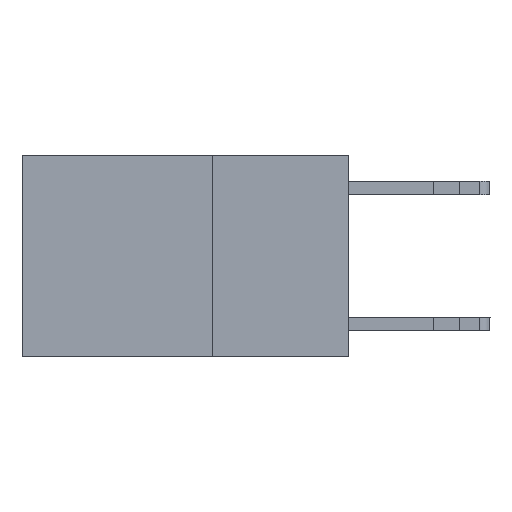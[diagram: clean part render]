
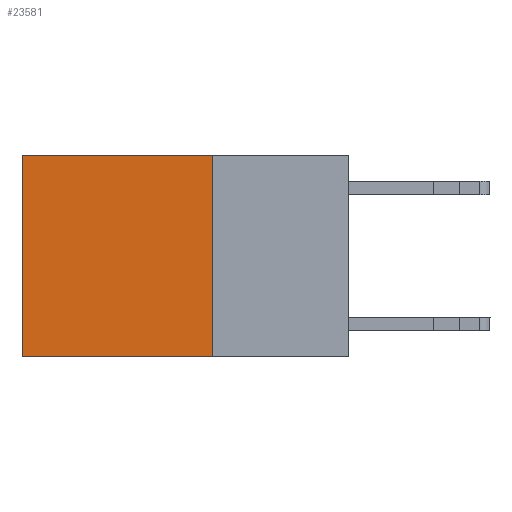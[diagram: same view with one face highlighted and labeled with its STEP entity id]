
A CAD part, left-side view. The second image highlights one B-rep face of the part: STEP entity #23581.
In plain terms, the highlighted planar face has unit normal (-1, 0, 0).
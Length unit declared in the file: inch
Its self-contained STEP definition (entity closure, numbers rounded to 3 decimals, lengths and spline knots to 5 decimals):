
#465 = EDGE_LOOP ( 'NONE', ( #22984, #8860, #528, #7988 ) ) ;
#528 = ORIENTED_EDGE ( 'NONE', *, *, #6625, .F. ) ;
#1226 = VERTEX_POINT ( 'NONE', #23646 ) ;
#1746 = FACE_OUTER_BOUND ( 'NONE', #465, .T. ) ;
#3121 = EDGE_CURVE ( 'NONE', #1226, #10511, #5561, .T. ) ;
#5373 = VECTOR ( 'NONE', #13706, 39.37008 ) ;
#5561 = LINE ( 'NONE', #11869, #5373 ) ;
#5748 = CARTESIAN_POINT ( 'NONE',  ( 0.2625, 0.6, -0.37 ) ) ;
#5767 = CARTESIAN_POINT ( 'NONE',  ( 0.2625, 0.25, 0. ) ) ;
#6070 = VECTOR ( 'NONE', #19828, 39.37008 ) ;
#6564 = VERTEX_POINT ( 'NONE', #21479 ) ;
#6625 = EDGE_CURVE ( 'NONE', #1226, #6564, #13777, .T. ) ;
#7526 = EDGE_CURVE ( 'NONE', #10511, #8958, #13548, .T. ) ;
#7988 = ORIENTED_EDGE ( 'NONE', *, *, #3121, .T. ) ;
#8051 = DIRECTION ( 'NONE',  ( 0., 1., 0. ) ) ;
#8632 = EDGE_CURVE ( 'NONE', #6564, #8958, #16431, .T. ) ;
#8860 = ORIENTED_EDGE ( 'NONE', *, *, #8632, .F. ) ;
#8958 = VERTEX_POINT ( 'NONE', #5748 ) ;
#9735 = DIRECTION ( 'NONE',  ( 1., 0., 0. ) ) ;
#10024 = CARTESIAN_POINT ( 'NONE',  ( 0.2625, 0.25, -0.37 ) ) ;
#10135 = CARTESIAN_POINT ( 'NONE',  ( 0.2625, 0.25, 0. ) ) ;
#10511 = VERTEX_POINT ( 'NONE', #24604 ) ;
#11869 = CARTESIAN_POINT ( 'NONE',  ( 0.2625, 0.25, 0. ) ) ;
#13548 = LINE ( 'NONE', #25554, #6070 ) ;
#13706 = DIRECTION ( 'NONE',  ( 0., 1., 0. ) ) ;
#13710 = VECTOR ( 'NONE', #25256, 39.37008 ) ;
#13777 = LINE ( 'NONE', #5767, #13710 ) ;
#15754 = AXIS2_PLACEMENT_3D ( 'NONE', #10135, #9735, #20211 ) ;
#16431 = LINE ( 'NONE', #10024, #22522 ) ;
#19828 = DIRECTION ( 'NONE',  ( 0., 0., -1. ) ) ;
#20211 = DIRECTION ( 'NONE',  ( 0., 0., -1. ) ) ;
#21479 = CARTESIAN_POINT ( 'NONE',  ( 0.2625, 0.25, -0.37 ) ) ;
#22522 = VECTOR ( 'NONE', #8051, 39.37008 ) ;
#22984 = ORIENTED_EDGE ( 'NONE', *, *, #7526, .T. ) ;
#23581 = ADVANCED_FACE ( 'NONE', ( #1746 ), #23733, .F. ) ;
#23646 = CARTESIAN_POINT ( 'NONE',  ( 0.2625, 0.25, 0. ) ) ;
#23733 = PLANE ( 'NONE',  #15754 ) ;
#24604 = CARTESIAN_POINT ( 'NONE',  ( 0.2625, 0.6, 0. ) ) ;
#25256 = DIRECTION ( 'NONE',  ( 0., 0., -1. ) ) ;
#25554 = CARTESIAN_POINT ( 'NONE',  ( 0.2625, 0.6, 0. ) ) ;
